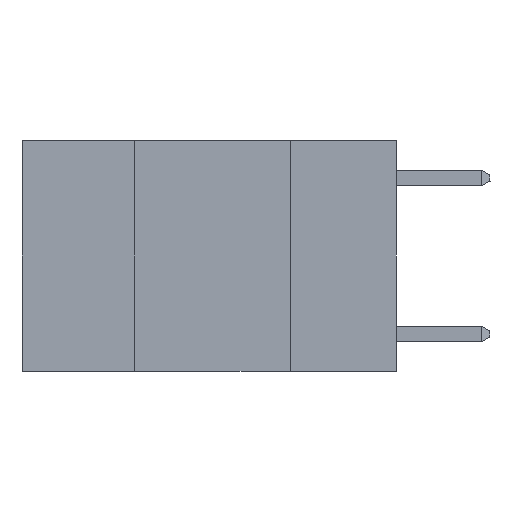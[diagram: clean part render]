
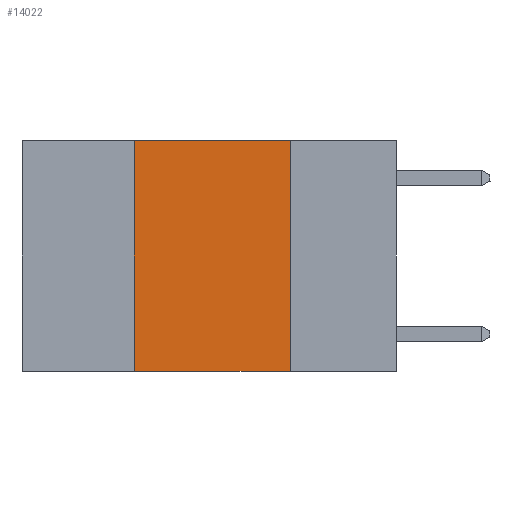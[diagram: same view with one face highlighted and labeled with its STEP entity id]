
A CAD part, left-side view. The second image highlights one B-rep face of the part: STEP entity #14022.
In plain terms, the highlighted planar face has unit normal (-1, 0, 0).
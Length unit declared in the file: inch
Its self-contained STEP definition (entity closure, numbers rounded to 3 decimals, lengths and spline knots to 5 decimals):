
#353 = LINE ( 'NONE', #1656, #15857 ) ;
#466 = VECTOR ( 'NONE', #24771, 39.37008 ) ;
#1108 = LINE ( 'NONE', #10736, #466 ) ;
#1656 = CARTESIAN_POINT ( 'NONE',  ( 0., 0.17, 0. ) ) ;
#2644 = CARTESIAN_POINT ( 'NONE',  ( 0., 0.6, 0. ) ) ;
#3545 = VERTEX_POINT ( 'NONE', #7713 ) ;
#3688 = DIRECTION ( 'NONE',  ( 0., 0., -1. ) ) ;
#3852 = CARTESIAN_POINT ( 'NONE',  ( 0., 0.42, 0. ) ) ;
#4237 = VERTEX_POINT ( 'NONE', #19772 ) ;
#4557 = PLANE ( 'NONE',  #13399 ) ;
#5706 = EDGE_LOOP ( 'NONE', ( #9048, #17592, #8467, #8860 ) ) ;
#6207 = VERTEX_POINT ( 'NONE', #24853 ) ;
#6577 = CARTESIAN_POINT ( 'NONE',  ( 0., 0.6, 0. ) ) ;
#7713 = CARTESIAN_POINT ( 'NONE',  ( 0., 0.17, -0.37 ) ) ;
#8046 = EDGE_CURVE ( 'NONE', #24744, #4237, #9036, .T. ) ;
#8467 = ORIENTED_EDGE ( 'NONE', *, *, #15066, .F. ) ;
#8637 = DIRECTION ( 'NONE',  ( 0., 0., -1. ) ) ;
#8860 = ORIENTED_EDGE ( 'NONE', *, *, #9933, .T. ) ;
#9036 = LINE ( 'NONE', #2644, #13771 ) ;
#9048 = ORIENTED_EDGE ( 'NONE', *, *, #22843, .F. ) ;
#9933 = EDGE_CURVE ( 'NONE', #6207, #3545, #13672, .T. ) ;
#10736 = CARTESIAN_POINT ( 'NONE',  ( 0., 0.42, 0. ) ) ;
#13399 = AXIS2_PLACEMENT_3D ( 'NONE', #6577, #20701, #8637 ) ;
#13672 = LINE ( 'NONE', #16269, #24322 ) ;
#13771 = VECTOR ( 'NONE', #14862, 39.37008 ) ;
#14022 = ADVANCED_FACE ( 'NONE', ( #18566 ), #4557, .F. ) ;
#14862 = DIRECTION ( 'NONE',  ( 0., -1., 0. ) ) ;
#15066 = EDGE_CURVE ( 'NONE', #6207, #24744, #1108, .T. ) ;
#15857 = VECTOR ( 'NONE', #3688, 39.37008 ) ;
#16269 = CARTESIAN_POINT ( 'NONE',  ( 0., 0.6, -0.37 ) ) ;
#17592 = ORIENTED_EDGE ( 'NONE', *, *, #8046, .F. ) ;
#18566 = FACE_OUTER_BOUND ( 'NONE', #5706, .T. ) ;
#19772 = CARTESIAN_POINT ( 'NONE',  ( 0., 0.17, 0. ) ) ;
#20701 = DIRECTION ( 'NONE',  ( 1., 0., 0. ) ) ;
#22305 = DIRECTION ( 'NONE',  ( 0., -1., 0. ) ) ;
#22843 = EDGE_CURVE ( 'NONE', #4237, #3545, #353, .T. ) ;
#24322 = VECTOR ( 'NONE', #22305, 39.37008 ) ;
#24744 = VERTEX_POINT ( 'NONE', #3852 ) ;
#24771 = DIRECTION ( 'NONE',  ( 0., 0., 1. ) ) ;
#24853 = CARTESIAN_POINT ( 'NONE',  ( 0., 0.42, -0.37 ) ) ;
